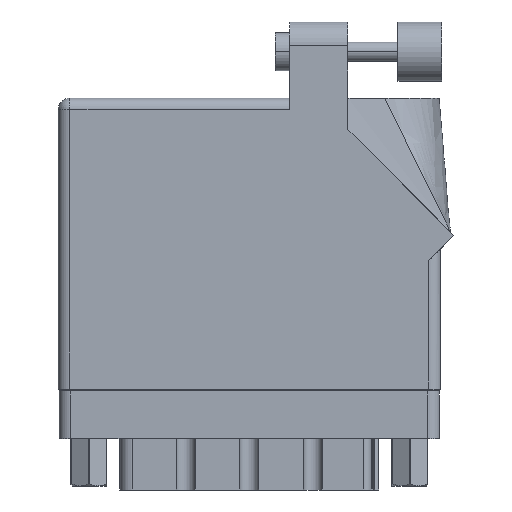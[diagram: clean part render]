
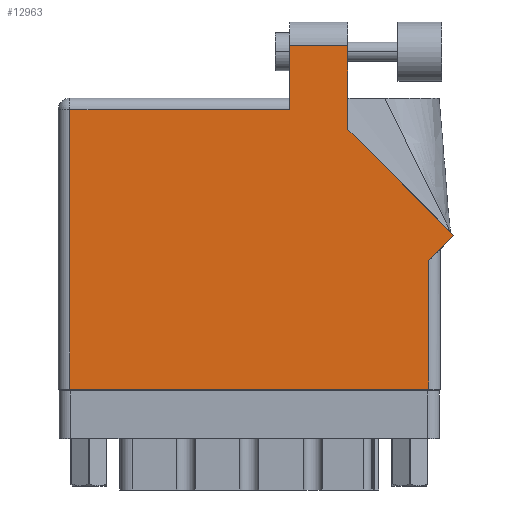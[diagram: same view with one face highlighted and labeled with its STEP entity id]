
A CAD part, front view. The second image highlights one B-rep face of the part: STEP entity #12963.
In plain terms, the highlighted face is planar.
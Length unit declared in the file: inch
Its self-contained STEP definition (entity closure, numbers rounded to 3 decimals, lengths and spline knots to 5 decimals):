
#1028 = DIRECTION ( 'NONE',  ( 0., -1., 0. ) ) ;
#2967 = VERTEX_POINT ( 'NONE', #13260 ) ;
#4385 = CARTESIAN_POINT ( 'NONE',  ( 1.948, 0., 0. ) ) ;
#4566 = CARTESIAN_POINT ( 'NONE',  ( 0.062, 0., 0. ) ) ;
#5693 = ORIENTED_EDGE ( 'NONE', *, *, #15845, .T. ) ;
#6511 = ORIENTED_EDGE ( 'NONE', *, *, #33766, .T. ) ;
#6743 = DIRECTION ( 'NONE',  ( 1., 0., 0. ) ) ;
#7137 = ORIENTED_EDGE ( 'NONE', *, *, #34694, .T. ) ;
#7584 = LINE ( 'NONE', #14647, #22044 ) ;
#8126 = PLANE ( 'NONE',  #26606 ) ;
#8252 = ORIENTED_EDGE ( 'NONE', *, *, #9013, .T. ) ;
#8393 = LINE ( 'NONE', #39483, #47691 ) ;
#9013 = EDGE_CURVE ( 'NONE', #35779, #14464, #9487, .T. ) ;
#9199 = VECTOR ( 'NONE', #44492, 39.37008 ) ;
#9487 = LINE ( 'NONE', #16480, #48138 ) ;
#10016 = LINE ( 'NONE', #35115, #23207 ) ;
#10234 = CARTESIAN_POINT ( 'NONE',  ( 1.524, 1.36442, 0. ) ) ;
#10877 = VERTEX_POINT ( 'NONE', #41068 ) ;
#11276 = ORIENTED_EDGE ( 'NONE', *, *, #11747, .T. ) ;
#11747 = EDGE_CURVE ( 'NONE', #10877, #47258, #27253, .T. ) ;
#12439 = VERTEX_POINT ( 'NONE', #32113 ) ;
#12963 = ADVANCED_FACE ( 'NONE', ( #22897 ), #8126, .F. ) ;
#13260 = CARTESIAN_POINT ( 'NONE',  ( 1.524, 1.805, 0. ) ) ;
#14272 = EDGE_LOOP ( 'NONE', ( #30900, #36663, #49035, #8252, #5693, #7137, #6511, #48173, #11276 ) ) ;
#14464 = VERTEX_POINT ( 'NONE', #15201 ) ;
#14647 = CARTESIAN_POINT ( 'NONE',  ( 0., 0., 0. ) ) ;
#15201 = CARTESIAN_POINT ( 'NONE',  ( 0.062, 1.468, 0. ) ) ;
#15845 = EDGE_CURVE ( 'NONE', #14464, #41239, #30249, .T. ) ;
#16357 = DIRECTION ( 'NONE',  ( 0.707, 0.707, 0. ) ) ;
#16480 = CARTESIAN_POINT ( 'NONE',  ( 0., 1.468, 0. ) ) ;
#17322 = VECTOR ( 'NONE', #44778, 39.37008 ) ;
#20940 = EDGE_CURVE ( 'NONE', #2967, #12439, #10016, .T. ) ;
#22044 = VECTOR ( 'NONE', #6743, 39.37008 ) ;
#22603 = LINE ( 'NONE', #40641, #32315 ) ;
#22897 = FACE_OUTER_BOUND ( 'NONE', #14272, .T. ) ;
#23207 = VECTOR ( 'NONE', #23777, 39.37008 ) ;
#23777 = DIRECTION ( 'NONE',  ( -1., 0., 0. ) ) ;
#26606 = AXIS2_PLACEMENT_3D ( 'NONE', #39492, #35097, #42908 ) ;
#27253 = LINE ( 'NONE', #36840, #9199 ) ;
#29366 = CARTESIAN_POINT ( 'NONE',  ( 1.217, 1.468, 0. ) ) ;
#30249 = LINE ( 'NONE', #38988, #31458 ) ;
#30900 = ORIENTED_EDGE ( 'NONE', *, *, #37858, .T. ) ;
#31458 = VECTOR ( 'NONE', #1028, 39.37008 ) ;
#32113 = CARTESIAN_POINT ( 'NONE',  ( 1.217, 1.805, 0. ) ) ;
#32315 = VECTOR ( 'NONE', #40471, 39.37008 ) ;
#33247 = CARTESIAN_POINT ( 'NONE',  ( 1.948, 0.737, 0. ) ) ;
#33766 = EDGE_CURVE ( 'NONE', #33944, #35247, #44536, .T. ) ;
#33944 = VERTEX_POINT ( 'NONE', #4385 ) ;
#34694 = EDGE_CURVE ( 'NONE', #41239, #33944, #7584, .T. ) ;
#35097 = DIRECTION ( 'NONE',  ( 0., 0., -1. ) ) ;
#35115 = CARTESIAN_POINT ( 'NONE',  ( 1.217, 1.805, 0. ) ) ;
#35247 = VERTEX_POINT ( 'NONE', #44860 ) ;
#35779 = VERTEX_POINT ( 'NONE', #29366 ) ;
#36663 = ORIENTED_EDGE ( 'NONE', *, *, #20940, .T. ) ;
#36840 = CARTESIAN_POINT ( 'NONE',  ( 2.08071, 0.80771, 0. ) ) ;
#37202 = VECTOR ( 'NONE', #41045, 39.37008 ) ;
#37273 = CARTESIAN_POINT ( 'NONE',  ( 1.524, 1.36442, 0. ) ) ;
#37858 = EDGE_CURVE ( 'NONE', #47258, #2967, #47505, .T. ) ;
#38406 = EDGE_CURVE ( 'NONE', #12439, #35779, #22603, .T. ) ;
#38988 = CARTESIAN_POINT ( 'NONE',  ( 0.062, 0., 0. ) ) ;
#39483 = CARTESIAN_POINT ( 'NONE',  ( 2.01, 0.737, 0. ) ) ;
#39492 = CARTESIAN_POINT ( 'NONE',  ( 0., 1.53, 0. ) ) ;
#40471 = DIRECTION ( 'NONE',  ( 0., -1., 0. ) ) ;
#40641 = CARTESIAN_POINT ( 'NONE',  ( 1.217, 1.53, 0. ) ) ;
#41045 = DIRECTION ( 'NONE',  ( 0., 1., 0. ) ) ;
#41068 = CARTESIAN_POINT ( 'NONE',  ( 2.08071, 0.80771, 0. ) ) ;
#41239 = VERTEX_POINT ( 'NONE', #4566 ) ;
#42908 = DIRECTION ( 'NONE',  ( -1., 0., 0. ) ) ;
#43537 = DIRECTION ( 'NONE',  ( -1., 0., 0. ) ) ;
#44492 = DIRECTION ( 'NONE',  ( -0.707, 0.707, 0. ) ) ;
#44536 = LINE ( 'NONE', #33247, #17322 ) ;
#44778 = DIRECTION ( 'NONE',  ( 0., 1., 0. ) ) ;
#44860 = CARTESIAN_POINT ( 'NONE',  ( 1.948, 0.675, 0. ) ) ;
#45564 = EDGE_CURVE ( 'NONE', #35247, #10877, #8393, .T. ) ;
#47258 = VERTEX_POINT ( 'NONE', #10234 ) ;
#47505 = LINE ( 'NONE', #37273, #37202 ) ;
#47691 = VECTOR ( 'NONE', #16357, 39.37008 ) ;
#48138 = VECTOR ( 'NONE', #43537, 39.37008 ) ;
#48173 = ORIENTED_EDGE ( 'NONE', *, *, #45564, .T. ) ;
#49035 = ORIENTED_EDGE ( 'NONE', *, *, #38406, .T. ) ;
